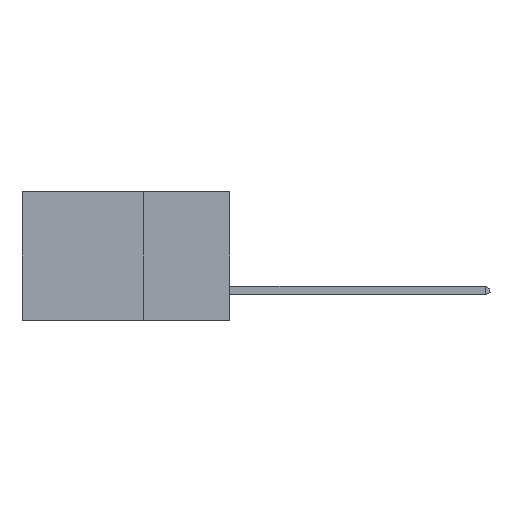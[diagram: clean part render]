
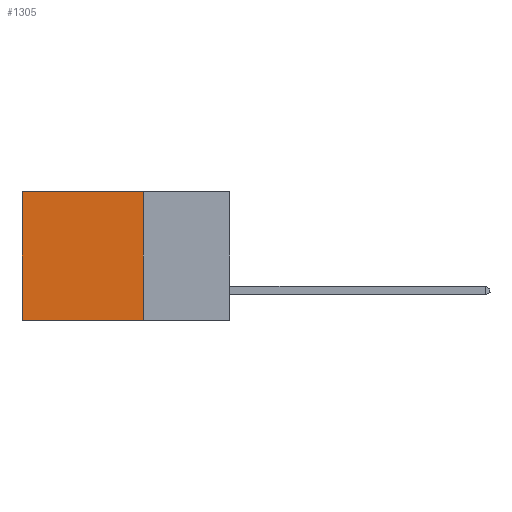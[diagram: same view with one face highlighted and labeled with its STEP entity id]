
A CAD part, left-side view. The second image highlights one B-rep face of the part: STEP entity #1305.
In plain terms, the highlighted planar face has unit normal (-1, 0, 0).
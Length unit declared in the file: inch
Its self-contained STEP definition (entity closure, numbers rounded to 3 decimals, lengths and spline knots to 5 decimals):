
#719 = DIRECTION ( 'NONE',  ( 1., 0., 0. ) ) ;
#1303 = FACE_OUTER_BOUND ( 'NONE', #1310, .T. ) ;
#1305 = ADVANCED_FACE ( 'NONE', ( #1303 ), #6460, .F. ) ;
#1310 = EDGE_LOOP ( 'NONE', ( #8668, #9766, #7817, #6113 ) ) ;
#1432 = DIRECTION ( 'NONE',  ( 0., 1., 0. ) ) ;
#1556 = CARTESIAN_POINT ( 'NONE',  ( 0.298, 0.25, 0. ) ) ;
#1898 = VECTOR ( 'NONE', #1432, 39.37008 ) ;
#2342 = CARTESIAN_POINT ( 'NONE',  ( 0.298, 0.25, -0.37 ) ) ;
#2415 = DIRECTION ( 'NONE',  ( 0., 0., -1. ) ) ;
#2840 = LINE ( 'NONE', #7522, #8451 ) ;
#3644 = LINE ( 'NONE', #7592, #11700 ) ;
#3852 = DIRECTION ( 'NONE',  ( 0., 0., -1. ) ) ;
#4030 = EDGE_CURVE ( 'NONE', #6942, #6229, #2840, .T. ) ;
#4261 = CARTESIAN_POINT ( 'NONE',  ( 0.298, 0.25, 0. ) ) ;
#4407 = LINE ( 'NONE', #4499, #7607 ) ;
#4499 = CARTESIAN_POINT ( 'NONE',  ( 0.298, 0.25, 0. ) ) ;
#4702 = VERTEX_POINT ( 'NONE', #10975 ) ;
#5283 = CARTESIAN_POINT ( 'NONE',  ( 0.298, 0.6, 0. ) ) ;
#5312 = EDGE_CURVE ( 'NONE', #11867, #4702, #11170, .T. ) ;
#5545 = DIRECTION ( 'NONE',  ( 0., 1., 0. ) ) ;
#6113 = ORIENTED_EDGE ( 'NONE', *, *, #4030, .T. ) ;
#6229 = VERTEX_POINT ( 'NONE', #5283 ) ;
#6460 = PLANE ( 'NONE',  #10936 ) ;
#6942 = VERTEX_POINT ( 'NONE', #4261 ) ;
#7522 = CARTESIAN_POINT ( 'NONE',  ( 0.298, 0.25, 0. ) ) ;
#7592 = CARTESIAN_POINT ( 'NONE',  ( 0.298, 0.6, 0. ) ) ;
#7607 = VECTOR ( 'NONE', #2415, 39.37008 ) ;
#7817 = ORIENTED_EDGE ( 'NONE', *, *, #7894, .F. ) ;
#7894 = EDGE_CURVE ( 'NONE', #6942, #11867, #4407, .T. ) ;
#8451 = VECTOR ( 'NONE', #5545, 39.37008 ) ;
#8668 = ORIENTED_EDGE ( 'NONE', *, *, #11893, .T. ) ;
#9553 = CARTESIAN_POINT ( 'NONE',  ( 0.298, 0.25, -0.37 ) ) ;
#9766 = ORIENTED_EDGE ( 'NONE', *, *, #5312, .F. ) ;
#10936 = AXIS2_PLACEMENT_3D ( 'NONE', #1556, #719, #11448 ) ;
#10975 = CARTESIAN_POINT ( 'NONE',  ( 0.298, 0.6, -0.37 ) ) ;
#11170 = LINE ( 'NONE', #2342, #1898 ) ;
#11448 = DIRECTION ( 'NONE',  ( 0., 0., -1. ) ) ;
#11700 = VECTOR ( 'NONE', #3852, 39.37008 ) ;
#11867 = VERTEX_POINT ( 'NONE', #9553 ) ;
#11893 = EDGE_CURVE ( 'NONE', #6229, #4702, #3644, .T. ) ;
